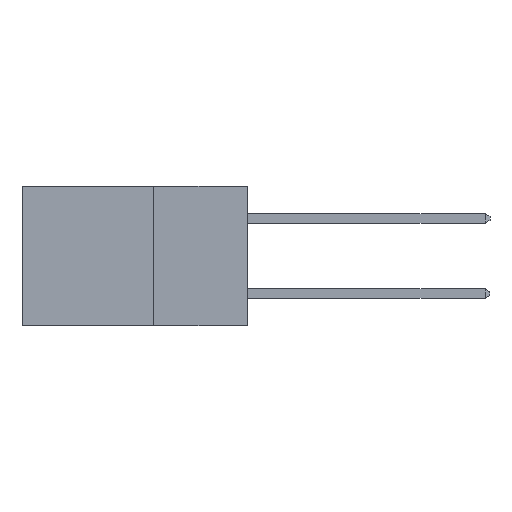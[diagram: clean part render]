
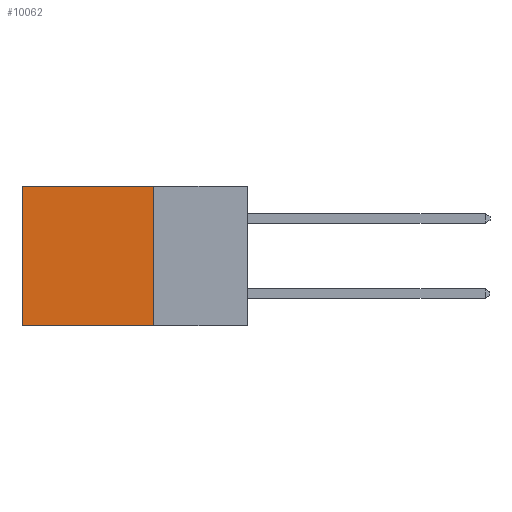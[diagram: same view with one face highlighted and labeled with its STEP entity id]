
A CAD part, left-side view. The second image highlights one B-rep face of the part: STEP entity #10062.
In plain terms, the highlighted planar face has unit normal (-1, 0, 0).
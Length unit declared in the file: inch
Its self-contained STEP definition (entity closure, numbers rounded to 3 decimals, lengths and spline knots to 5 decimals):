
#310 = LINE ( 'NONE', #3339, #1767 ) ;
#385 = EDGE_CURVE ( 'NONE', #14167, #6875, #2454, .T. ) ;
#411 = AXIS2_PLACEMENT_3D ( 'NONE', #6282, #6336, #14168 ) ;
#645 = LINE ( 'NONE', #5688, #11690 ) ;
#784 = VECTOR ( 'NONE', #6995, 39.37008 ) ;
#1336 = CARTESIAN_POINT ( 'NONE',  ( 0.298, 0.25, 0. ) ) ;
#1767 = VECTOR ( 'NONE', #6492, 39.37008 ) ;
#2454 = LINE ( 'NONE', #9766, #11130 ) ;
#3339 = CARTESIAN_POINT ( 'NONE',  ( 0.298, 0.6, 0. ) ) ;
#3850 = EDGE_CURVE ( 'NONE', #6875, #9861, #310, .T. ) ;
#3852 = LINE ( 'NONE', #1336, #784 ) ;
#5418 = DIRECTION ( 'NONE',  ( 0., 1., 0. ) ) ;
#5688 = CARTESIAN_POINT ( 'NONE',  ( 0.298, 0.25, -0.37 ) ) ;
#5939 = EDGE_LOOP ( 'NONE', ( #6386, #7429, #7993, #12646 ) ) ;
#6282 = CARTESIAN_POINT ( 'NONE',  ( 0.298, 0.25, 0. ) ) ;
#6336 = DIRECTION ( 'NONE',  ( 1., 0., 0. ) ) ;
#6386 = ORIENTED_EDGE ( 'NONE', *, *, #3850, .T. ) ;
#6492 = DIRECTION ( 'NONE',  ( 0., 0., -1. ) ) ;
#6649 = VERTEX_POINT ( 'NONE', #12424 ) ;
#6875 = VERTEX_POINT ( 'NONE', #8316 ) ;
#6995 = DIRECTION ( 'NONE',  ( 0., 0., -1. ) ) ;
#7052 = EDGE_CURVE ( 'NONE', #6649, #9861, #645, .T. ) ;
#7095 = CARTESIAN_POINT ( 'NONE',  ( 0.298, 0.6, -0.37 ) ) ;
#7429 = ORIENTED_EDGE ( 'NONE', *, *, #7052, .F. ) ;
#7507 = DIRECTION ( 'NONE',  ( 0., 1., 0. ) ) ;
#7993 = ORIENTED_EDGE ( 'NONE', *, *, #14366, .F. ) ;
#8316 = CARTESIAN_POINT ( 'NONE',  ( 0.298, 0.6, 0. ) ) ;
#9766 = CARTESIAN_POINT ( 'NONE',  ( 0.298, 0.25, 0. ) ) ;
#9861 = VERTEX_POINT ( 'NONE', #7095 ) ;
#10062 = ADVANCED_FACE ( 'NONE', ( #11438 ), #13048, .F. ) ;
#11130 = VECTOR ( 'NONE', #7507, 39.37008 ) ;
#11438 = FACE_OUTER_BOUND ( 'NONE', #5939, .T. ) ;
#11690 = VECTOR ( 'NONE', #5418, 39.37008 ) ;
#12424 = CARTESIAN_POINT ( 'NONE',  ( 0.298, 0.25, -0.37 ) ) ;
#12646 = ORIENTED_EDGE ( 'NONE', *, *, #385, .T. ) ;
#13048 = PLANE ( 'NONE',  #411 ) ;
#14167 = VERTEX_POINT ( 'NONE', #14420 ) ;
#14168 = DIRECTION ( 'NONE',  ( 0., 0., -1. ) ) ;
#14366 = EDGE_CURVE ( 'NONE', #14167, #6649, #3852, .T. ) ;
#14420 = CARTESIAN_POINT ( 'NONE',  ( 0.298, 0.25, 0. ) ) ;
